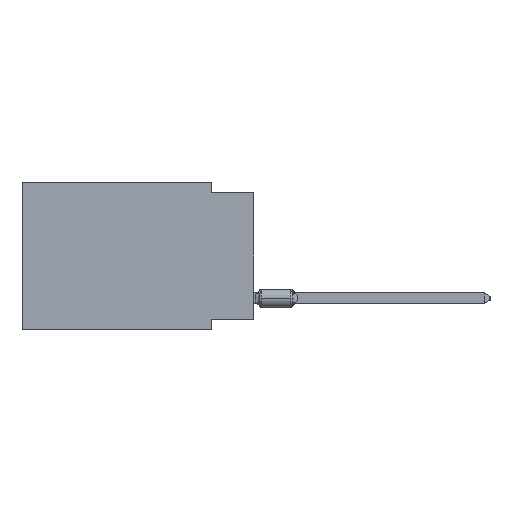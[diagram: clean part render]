
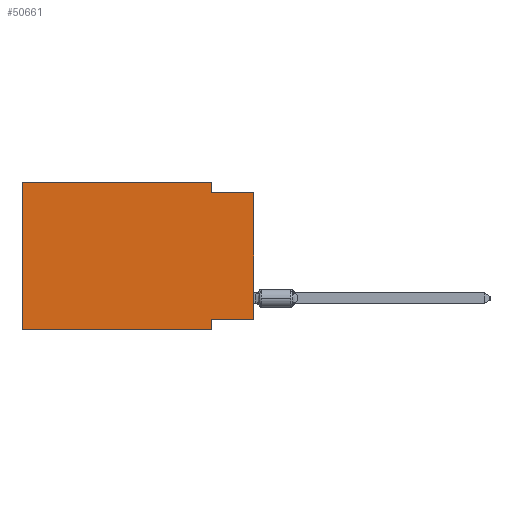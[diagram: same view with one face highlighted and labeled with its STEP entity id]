
A CAD part, left-side view. The second image highlights one B-rep face of the part: STEP entity #50661.
In plain terms, the highlighted planar face has unit normal (-1, 0, 0).
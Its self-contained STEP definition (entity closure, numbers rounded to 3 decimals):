
#184 = DIRECTION ( 'NONE',  ( 0., 0., -1. ) ) ;
#306 = CARTESIAN_POINT ( 'NONE',  ( 0., 2.54, -8.255 ) ) ;
#1746 = VECTOR ( 'NONE', #34822, 1000. ) ;
#2113 = VECTOR ( 'NONE', #53345, 1000. ) ;
#2868 = CARTESIAN_POINT ( 'NONE',  ( 0., 2.54, 0. ) ) ;
#3226 = DIRECTION ( 'NONE',  ( 0., -1., 0. ) ) ;
#4414 = VERTEX_POINT ( 'NONE', #306 ) ;
#5333 = CARTESIAN_POINT ( 'NONE',  ( 0., 13.97, 0. ) ) ;
#6173 = LINE ( 'NONE', #35700, #2113 ) ;
#6367 = EDGE_CURVE ( 'NONE', #11756, #10381, #7139, .T. ) ;
#7124 = DIRECTION ( 'NONE',  ( 0., 0., 1. ) ) ;
#7139 = LINE ( 'NONE', #56018, #44270 ) ;
#9101 = ORIENTED_EDGE ( 'NONE', *, *, #6367, .F. ) ;
#10381 = VERTEX_POINT ( 'NONE', #32365 ) ;
#10707 = VERTEX_POINT ( 'NONE', #49679 ) ;
#11353 = ORIENTED_EDGE ( 'NONE', *, *, #56780, .T. ) ;
#11471 = DIRECTION ( 'NONE',  ( 0., 0., -1. ) ) ;
#11756 = VERTEX_POINT ( 'NONE', #2868 ) ;
#12080 = CARTESIAN_POINT ( 'NONE',  ( 0., 0., -8.255 ) ) ;
#12174 = LINE ( 'NONE', #42841, #54171 ) ;
#14423 = CARTESIAN_POINT ( 'NONE',  ( 0., 13.97, -8.89 ) ) ;
#14979 = LINE ( 'NONE', #14423, #22392 ) ;
#15288 = DIRECTION ( 'NONE',  ( 0., 1., 0. ) ) ;
#16951 = VECTOR ( 'NONE', #7124, 1000. ) ;
#17182 = CARTESIAN_POINT ( 'NONE',  ( 0., 13.97, 0. ) ) ;
#18772 = DIRECTION ( 'NONE',  ( 0., -1., 0. ) ) ;
#19665 = ORIENTED_EDGE ( 'NONE', *, *, #29882, .T. ) ;
#20589 = ORIENTED_EDGE ( 'NONE', *, *, #28290, .F. ) ;
#22392 = VECTOR ( 'NONE', #49710, 1000. ) ;
#23283 = CARTESIAN_POINT ( 'NONE',  ( 0., 2.54, -8.89 ) ) ;
#23610 = AXIS2_PLACEMENT_3D ( 'NONE', #48188, #43855, #184 ) ;
#23804 = VERTEX_POINT ( 'NONE', #49854 ) ;
#28098 = VECTOR ( 'NONE', #18772, 1000. ) ;
#28290 = EDGE_CURVE ( 'NONE', #34153, #4414, #46227, .T. ) ;
#28301 = ORIENTED_EDGE ( 'NONE', *, *, #40189, .F. ) ;
#29243 = ORIENTED_EDGE ( 'NONE', *, *, #33129, .F. ) ;
#29882 = EDGE_CURVE ( 'NONE', #34153, #23804, #42992, .T. ) ;
#30145 = VERTEX_POINT ( 'NONE', #23283 ) ;
#32365 = CARTESIAN_POINT ( 'NONE',  ( 0., 2.54, -0.635 ) ) ;
#33129 = EDGE_CURVE ( 'NONE', #40103, #11756, #12174, .T. ) ;
#33994 = EDGE_CURVE ( 'NONE', #10707, #40103, #39148, .T. ) ;
#34153 = VERTEX_POINT ( 'NONE', #55293 ) ;
#34822 = DIRECTION ( 'NONE',  ( 0., 0., 1. ) ) ;
#35700 = CARTESIAN_POINT ( 'NONE',  ( 0., 2.54, -8.89 ) ) ;
#39148 = LINE ( 'NONE', #17182, #1746 ) ;
#40103 = VERTEX_POINT ( 'NONE', #5333 ) ;
#40189 = EDGE_CURVE ( 'NONE', #4414, #30145, #6173, .T. ) ;
#41056 = CARTESIAN_POINT ( 'NONE',  ( 0., 0., -0.635 ) ) ;
#42841 = CARTESIAN_POINT ( 'NONE',  ( 0., 13.97, 0. ) ) ;
#42992 = LINE ( 'NONE', #46751, #16951 ) ;
#43265 = PLANE ( 'NONE',  #23610 ) ;
#43855 = DIRECTION ( 'NONE',  ( 1., 0., 0. ) ) ;
#44270 = VECTOR ( 'NONE', #11471, 1000. ) ;
#45578 = VECTOR ( 'NONE', #15288, 1000. ) ;
#46227 = LINE ( 'NONE', #12080, #45578 ) ;
#46751 = CARTESIAN_POINT ( 'NONE',  ( 0., 0., 0. ) ) ;
#48188 = CARTESIAN_POINT ( 'NONE',  ( 0., 13.97, 0. ) ) ;
#49065 = ORIENTED_EDGE ( 'NONE', *, *, #49950, .F. ) ;
#49073 = EDGE_LOOP ( 'NONE', ( #19665, #49065, #9101, #29243, #49781, #11353, #28301, #20589 ) ) ;
#49679 = CARTESIAN_POINT ( 'NONE',  ( 0., 13.97, -8.89 ) ) ;
#49710 = DIRECTION ( 'NONE',  ( 0., -1., 0. ) ) ;
#49781 = ORIENTED_EDGE ( 'NONE', *, *, #33994, .F. ) ;
#49854 = CARTESIAN_POINT ( 'NONE',  ( 0., 0., -0.635 ) ) ;
#49950 = EDGE_CURVE ( 'NONE', #10381, #23804, #54080, .T. ) ;
#50661 = ADVANCED_FACE ( 'NONE', ( #51944 ), #43265, .F. ) ;
#51944 = FACE_OUTER_BOUND ( 'NONE', #49073, .T. ) ;
#53345 = DIRECTION ( 'NONE',  ( 0., 0., -1. ) ) ;
#54080 = LINE ( 'NONE', #41056, #28098 ) ;
#54171 = VECTOR ( 'NONE', #3226, 1000. ) ;
#55293 = CARTESIAN_POINT ( 'NONE',  ( 0., 0., -8.255 ) ) ;
#56018 = CARTESIAN_POINT ( 'NONE',  ( 0., 2.54, 0. ) ) ;
#56780 = EDGE_CURVE ( 'NONE', #10707, #30145, #14979, .T. ) ;
